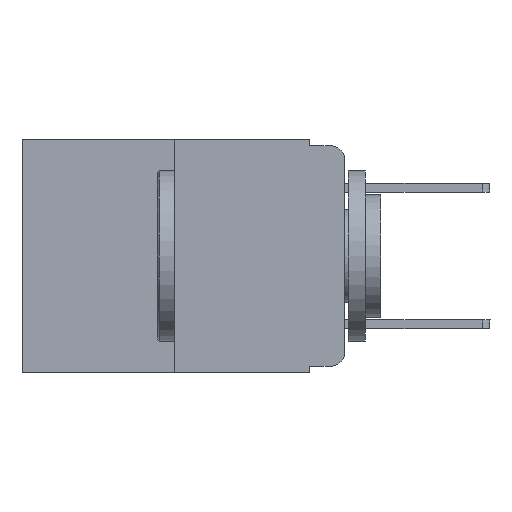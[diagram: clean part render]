
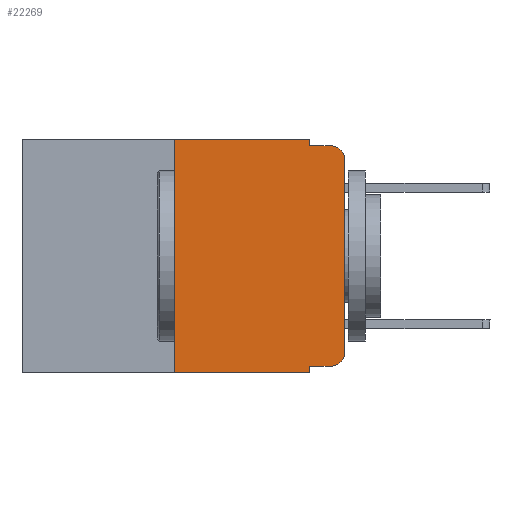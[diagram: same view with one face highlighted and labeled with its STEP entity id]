
A CAD part, left-side view. The second image highlights one B-rep face of the part: STEP entity #22269.
In plain terms, the highlighted planar face has unit normal (-1, 0, 0).
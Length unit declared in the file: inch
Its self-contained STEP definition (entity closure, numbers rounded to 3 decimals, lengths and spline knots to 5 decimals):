
#681 = ORIENTED_EDGE ( 'NONE', *, *, #6865, .T. ) ;
#947 = VERTEX_POINT ( 'NONE', #10500 ) ;
#1159 = CARTESIAN_POINT ( 'NONE',  ( 0., 0.051, -0.333 ) ) ;
#1284 = ORIENTED_EDGE ( 'NONE', *, *, #21754, .F. ) ;
#1830 = DIRECTION ( 'NONE',  ( 0., 0., -1. ) ) ;
#1923 = VECTOR ( 'NONE', #19169, 39.37008 ) ;
#2253 = VERTEX_POINT ( 'NONE', #8577 ) ;
#2603 = VERTEX_POINT ( 'NONE', #17303 ) ;
#2765 = LINE ( 'NONE', #4478, #1923 ) ;
#2976 = CARTESIAN_POINT ( 'NONE',  ( 0., 0.051, 0. ) ) ;
#3585 = CARTESIAN_POINT ( 'NONE',  ( 0., 0.051, 0. ) ) ;
#3845 = ORIENTED_EDGE ( 'NONE', *, *, #9817, .F. ) ;
#4290 = CARTESIAN_POINT ( 'NONE',  ( 0., 0.473, 0. ) ) ;
#4478 = CARTESIAN_POINT ( 'NONE',  ( 0., 0.473, -0.343 ) ) ;
#4619 = ORIENTED_EDGE ( 'NONE', *, *, #12683, .F. ) ;
#4631 = FACE_OUTER_BOUND ( 'NONE', #6819, .T. ) ;
#4639 = LINE ( 'NONE', #16086, #18150 ) ;
#4656 = VECTOR ( 'NONE', #5865, 39.37008 ) ;
#4758 = CARTESIAN_POINT ( 'NONE',  ( 0., 0.473, 0. ) ) ;
#4813 = CARTESIAN_POINT ( 'NONE',  ( 0., 0.051, -0.01 ) ) ;
#4980 = LINE ( 'NONE', #12062, #22700 ) ;
#5099 = DIRECTION ( 'NONE',  ( 0., 0., 1. ) ) ;
#5156 = EDGE_CURVE ( 'NONE', #16660, #17525, #2765, .T. ) ;
#5675 = DIRECTION ( 'NONE',  ( -1., 0., 0. ) ) ;
#5865 = DIRECTION ( 'NONE',  ( 0., -1., 0. ) ) ;
#6819 = EDGE_LOOP ( 'NONE', ( #681, #8831, #4619, #10498, #1284, #3845, #17632, #7727, #16364, #23571 ) ) ;
#6820 = DIRECTION ( 'NONE',  ( 0., -1., 0. ) ) ;
#6865 = EDGE_CURVE ( 'NONE', #22320, #2603, #4639, .T. ) ;
#7186 = LINE ( 'NONE', #3585, #18470 ) ;
#7452 = EDGE_CURVE ( 'NONE', #11391, #17525, #7186, .T. ) ;
#7727 = ORIENTED_EDGE ( 'NONE', *, *, #7452, .F. ) ;
#8061 = CARTESIAN_POINT ( 'NONE',  ( 0., 0.051, -0.333 ) ) ;
#8158 = DIRECTION ( 'NONE',  ( 0., 0., -1. ) ) ;
#8365 = EDGE_CURVE ( 'NONE', #11391, #12806, #11701, .T. ) ;
#8577 = CARTESIAN_POINT ( 'NONE',  ( 0., 0.02, -0.01 ) ) ;
#8831 = ORIENTED_EDGE ( 'NONE', *, *, #21195, .T. ) ;
#9167 = CARTESIAN_POINT ( 'NONE',  ( 0., 0.02, -0.03 ) ) ;
#9590 = LINE ( 'NONE', #4290, #4656 ) ;
#9817 = EDGE_CURVE ( 'NONE', #16660, #947, #4980, .T. ) ;
#10498 = ORIENTED_EDGE ( 'NONE', *, *, #10752, .F. ) ;
#10500 = CARTESIAN_POINT ( 'NONE',  ( 0., 0.25, 0. ) ) ;
#10752 = EDGE_CURVE ( 'NONE', #20238, #17823, #13734, .T. ) ;
#11136 = VECTOR ( 'NONE', #20641, 39.37008 ) ;
#11262 = CARTESIAN_POINT ( 'NONE',  ( 0., 0.02, -0.333 ) ) ;
#11335 = DIRECTION ( 'NONE',  ( 0., 0., -1. ) ) ;
#11391 = VERTEX_POINT ( 'NONE', #1159 ) ;
#11701 = LINE ( 'NONE', #8061, #11136 ) ;
#11951 = CARTESIAN_POINT ( 'NONE',  ( 0., 0.25, -0.343 ) ) ;
#11955 = PLANE ( 'NONE',  #18506 ) ;
#12062 = CARTESIAN_POINT ( 'NONE',  ( 0., 0.25, 0. ) ) ;
#12076 = DIRECTION ( 'NONE',  ( 0., 0., -1. ) ) ;
#12088 = DIRECTION ( 'NONE',  ( 0., 0., 1. ) ) ;
#12683 = EDGE_CURVE ( 'NONE', #17823, #2253, #21313, .T. ) ;
#12806 = VERTEX_POINT ( 'NONE', #11262 ) ;
#13413 = CIRCLE ( 'NONE', #18426, 0.02 ) ;
#13734 = LINE ( 'NONE', #15314, #18079 ) ;
#14706 = VECTOR ( 'NONE', #6820, 39.37008 ) ;
#14937 = DIRECTION ( 'NONE',  ( 0., 0., -1. ) ) ;
#14978 = CARTESIAN_POINT ( 'NONE',  ( 0., 0.02, -0.313 ) ) ;
#15135 = CARTESIAN_POINT ( 'NONE',  ( 0., 0.051, -0.01 ) ) ;
#15314 = CARTESIAN_POINT ( 'NONE',  ( 0., 0.051, 0. ) ) ;
#16086 = CARTESIAN_POINT ( 'NONE',  ( 0., 0., 0. ) ) ;
#16364 = ORIENTED_EDGE ( 'NONE', *, *, #8365, .T. ) ;
#16660 = VERTEX_POINT ( 'NONE', #11951 ) ;
#17303 = CARTESIAN_POINT ( 'NONE',  ( 0., 0., -0.03 ) ) ;
#17525 = VERTEX_POINT ( 'NONE', #19476 ) ;
#17632 = ORIENTED_EDGE ( 'NONE', *, *, #5156, .T. ) ;
#17823 = VERTEX_POINT ( 'NONE', #15135 ) ;
#18079 = VECTOR ( 'NONE', #8158, 39.37008 ) ;
#18150 = VECTOR ( 'NONE', #12088, 39.37008 ) ;
#18426 = AXIS2_PLACEMENT_3D ( 'NONE', #14978, #5675, #1830 ) ;
#18470 = VECTOR ( 'NONE', #14937, 39.37008 ) ;
#18506 = AXIS2_PLACEMENT_3D ( 'NONE', #4758, #22720, #12076 ) ;
#19169 = DIRECTION ( 'NONE',  ( 0., -1., 0. ) ) ;
#19476 = CARTESIAN_POINT ( 'NONE',  ( 0., 0.051, -0.343 ) ) ;
#20028 = CIRCLE ( 'NONE', #21905, 0.02 ) ;
#20238 = VERTEX_POINT ( 'NONE', #2976 ) ;
#20277 = DIRECTION ( 'NONE',  ( -1., 0., 0. ) ) ;
#20641 = DIRECTION ( 'NONE',  ( 0., -1., 0. ) ) ;
#21028 = CARTESIAN_POINT ( 'NONE',  ( 0., 0., -0.313 ) ) ;
#21183 = EDGE_CURVE ( 'NONE', #12806, #22320, #13413, .T. ) ;
#21195 = EDGE_CURVE ( 'NONE', #2603, #2253, #20028, .T. ) ;
#21313 = LINE ( 'NONE', #4813, #14706 ) ;
#21754 = EDGE_CURVE ( 'NONE', #947, #20238, #9590, .T. ) ;
#21905 = AXIS2_PLACEMENT_3D ( 'NONE', #9167, #20277, #11335 ) ;
#22269 = ADVANCED_FACE ( 'NONE', ( #4631 ), #11955, .F. ) ;
#22320 = VERTEX_POINT ( 'NONE', #21028 ) ;
#22700 = VECTOR ( 'NONE', #5099, 39.37008 ) ;
#22720 = DIRECTION ( 'NONE',  ( 1., 0., 0. ) ) ;
#23571 = ORIENTED_EDGE ( 'NONE', *, *, #21183, .T. ) ;
